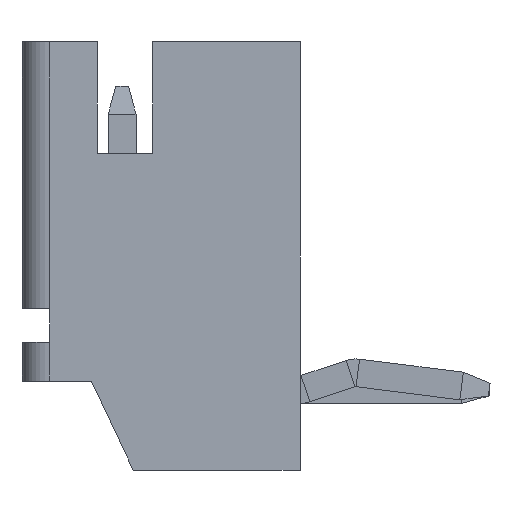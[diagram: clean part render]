
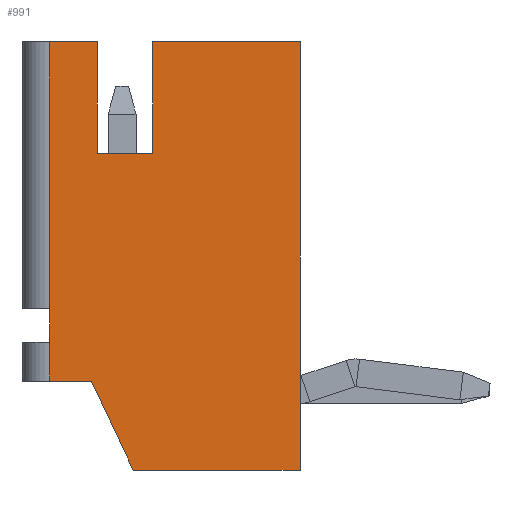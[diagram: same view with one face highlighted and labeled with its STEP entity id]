
A CAD part, left-side view. The second image highlights one B-rep face of the part: STEP entity #991.
In plain terms, the highlighted planar face has unit normal (-1, 0, 0).
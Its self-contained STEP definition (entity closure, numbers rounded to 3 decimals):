
#13 = CARTESIAN_POINT ( 'NONE',  ( -2., 1.3, 0. ) ) ;
#51 = VECTOR ( 'NONE', #4264, 1000. ) ;
#98 = CARTESIAN_POINT ( 'NONE',  ( -2., 1.3, 1.3 ) ) ;
#130 = EDGE_CURVE ( 'NONE', #6162, #6657, #4499, .T. ) ;
#144 = VERTEX_POINT ( 'NONE', #475 ) ;
#177 = CARTESIAN_POINT ( 'NONE',  ( -2., -3.2, -1.6 ) ) ;
#223 = ORIENTED_EDGE ( 'NONE', *, *, #1358, .T. ) ;
#278 = VECTOR ( 'NONE', #2242, 1000. ) ;
#312 = CARTESIAN_POINT ( 'NONE',  ( -2., 1.3, 6.1 ) ) ;
#313 = CARTESIAN_POINT ( 'NONE',  ( -2., 1.3, 1.3 ) ) ;
#388 = EDGE_LOOP ( 'NONE', ( #1018, #1633, #5628, #573, #6049, #5959, #5366, #223, #3068, #3339, #4665, #1681 ) ) ;
#448 = EDGE_CURVE ( 'NONE', #1024, #3373, #1513, .T. ) ;
#475 = CARTESIAN_POINT ( 'NONE',  ( -2., 0.55, 0. ) ) ;
#573 = ORIENTED_EDGE ( 'NONE', *, *, #1032, .T. ) ;
#593 = CARTESIAN_POINT ( 'NONE',  ( -2., 1.3, 0. ) ) ;
#616 = DIRECTION ( 'NONE',  ( 0., 0., -1. ) ) ;
#653 = CARTESIAN_POINT ( 'NONE',  ( -2., -3.2, 6.1 ) ) ;
#654 = CARTESIAN_POINT ( 'NONE',  ( -2., 1.3, 0.7 ) ) ;
#693 = VECTOR ( 'NONE', #4263, 1000. ) ;
#991 = ADVANCED_FACE ( 'NONE', ( #5384 ), #5811, .T. ) ;
#1018 = ORIENTED_EDGE ( 'NONE', *, *, #2460, .T. ) ;
#1024 = VERTEX_POINT ( 'NONE', #177 ) ;
#1032 = EDGE_CURVE ( 'NONE', #144, #1546, #3606, .T. ) ;
#1115 = VECTOR ( 'NONE', #4143, 1000. ) ;
#1137 = DIRECTION ( 'NONE',  ( -1., 0., 0. ) ) ;
#1193 = CARTESIAN_POINT ( 'NONE',  ( -2., 0.45, 4.1 ) ) ;
#1358 = EDGE_CURVE ( 'NONE', #1372, #6162, #3042, .T. ) ;
#1372 = VERTEX_POINT ( 'NONE', #2681 ) ;
#1513 = LINE ( 'NONE', #3240, #51 ) ;
#1518 = VECTOR ( 'NONE', #3710, 1000. ) ;
#1546 = VERTEX_POINT ( 'NONE', #2281 ) ;
#1588 = EDGE_CURVE ( 'NONE', #5779, #4288, #2639, .T. ) ;
#1633 = ORIENTED_EDGE ( 'NONE', *, *, #1588, .T. ) ;
#1656 = LINE ( 'NONE', #3238, #278 ) ;
#1678 = CARTESIAN_POINT ( 'NONE',  ( -2., -0.55, 6.1 ) ) ;
#1681 = ORIENTED_EDGE ( 'NONE', *, *, #1809, .T. ) ;
#1741 = DIRECTION ( 'NONE',  ( 0., -1., 0. ) ) ;
#1809 = EDGE_CURVE ( 'NONE', #3515, #5945, #3206, .T. ) ;
#1899 = CARTESIAN_POINT ( 'NONE',  ( -2., -0.55, 4.1 ) ) ;
#2242 = DIRECTION ( 'NONE',  ( 0., 1., 0. ) ) ;
#2281 = CARTESIAN_POINT ( 'NONE',  ( -2., -0.2, -1.6 ) ) ;
#2403 = DIRECTION ( 'NONE',  ( 0., 0., -1. ) ) ;
#2460 = EDGE_CURVE ( 'NONE', #5945, #5779, #3911, .T. ) ;
#2543 = VECTOR ( 'NONE', #3811, 1000. ) ;
#2548 = VECTOR ( 'NONE', #1741, 1000. ) ;
#2596 = DIRECTION ( 'NONE',  ( 0., 0., -1. ) ) ;
#2639 = LINE ( 'NONE', #2905, #5448 ) ;
#2681 = CARTESIAN_POINT ( 'NONE',  ( -2., -0.55, 6.1 ) ) ;
#2745 = DIRECTION ( 'NONE',  ( 0., -1., 0. ) ) ;
#2905 = CARTESIAN_POINT ( 'NONE',  ( -2., 1.3, 0. ) ) ;
#2951 = LINE ( 'NONE', #1678, #693 ) ;
#2964 = VECTOR ( 'NONE', #2596, 1000. ) ;
#3042 = LINE ( 'NONE', #4677, #6099 ) ;
#3068 = ORIENTED_EDGE ( 'NONE', *, *, #130, .T. ) ;
#3205 = CARTESIAN_POINT ( 'NONE',  ( -2., 1.8, 0. ) ) ;
#3206 = LINE ( 'NONE', #593, #2964 ) ;
#3238 = CARTESIAN_POINT ( 'NONE',  ( -2., 1.8, 6.1 ) ) ;
#3240 = CARTESIAN_POINT ( 'NONE',  ( -2., -3.2, 6.1 ) ) ;
#3339 = ORIENTED_EDGE ( 'NONE', *, *, #5858, .T. ) ;
#3373 = VERTEX_POINT ( 'NONE', #653 ) ;
#3515 = VERTEX_POINT ( 'NONE', #312 ) ;
#3606 = LINE ( 'NONE', #6324, #1518 ) ;
#3638 = DIRECTION ( 'NONE',  ( 0., -1., 0. ) ) ;
#3710 = DIRECTION ( 'NONE',  ( 0., -0.424, -0.905 ) ) ;
#3811 = DIRECTION ( 'NONE',  ( 0., 0., 1. ) ) ;
#3901 = LINE ( 'NONE', #5809, #2543 ) ;
#3911 = LINE ( 'NONE', #98, #4147 ) ;
#4064 = LINE ( 'NONE', #3205, #2548 ) ;
#4077 = CARTESIAN_POINT ( 'NONE',  ( -2., 0.45, 4.1 ) ) ;
#4143 = DIRECTION ( 'NONE',  ( 0., 1., 0. ) ) ;
#4147 = VECTOR ( 'NONE', #616, 1000. ) ;
#4180 = VERTEX_POINT ( 'NONE', #6006 ) ;
#4214 = CARTESIAN_POINT ( 'NONE',  ( -2., 0., 0. ) ) ;
#4263 = DIRECTION ( 'NONE',  ( 0., 1., 0. ) ) ;
#4264 = DIRECTION ( 'NONE',  ( 0., 0., 1. ) ) ;
#4288 = VERTEX_POINT ( 'NONE', #13 ) ;
#4368 = EDGE_CURVE ( 'NONE', #4288, #144, #4064, .T. ) ;
#4387 = VECTOR ( 'NONE', #3638, 1000. ) ;
#4499 = LINE ( 'NONE', #4077, #1115 ) ;
#4548 = AXIS2_PLACEMENT_3D ( 'NONE', #4214, #1137, #2745 ) ;
#4635 = LINE ( 'NONE', #4639, #4387 ) ;
#4639 = CARTESIAN_POINT ( 'NONE',  ( -2., -3.2, -1.6 ) ) ;
#4665 = ORIENTED_EDGE ( 'NONE', *, *, #5837, .T. ) ;
#4677 = CARTESIAN_POINT ( 'NONE',  ( -2., -0.55, 6.1 ) ) ;
#4732 = EDGE_CURVE ( 'NONE', #3373, #1372, #2951, .T. ) ;
#5366 = ORIENTED_EDGE ( 'NONE', *, *, #4732, .T. ) ;
#5384 = FACE_OUTER_BOUND ( 'NONE', #388, .T. ) ;
#5448 = VECTOR ( 'NONE', #2403, 1000. ) ;
#5480 = EDGE_CURVE ( 'NONE', #1546, #1024, #4635, .T. ) ;
#5628 = ORIENTED_EDGE ( 'NONE', *, *, #4368, .T. ) ;
#5779 = VERTEX_POINT ( 'NONE', #654 ) ;
#5809 = CARTESIAN_POINT ( 'NONE',  ( -2., 0.45, 6.1 ) ) ;
#5811 = PLANE ( 'NONE',  #4548 ) ;
#5837 = EDGE_CURVE ( 'NONE', #4180, #3515, #1656, .T. ) ;
#5858 = EDGE_CURVE ( 'NONE', #6657, #4180, #3901, .T. ) ;
#5945 = VERTEX_POINT ( 'NONE', #313 ) ;
#5959 = ORIENTED_EDGE ( 'NONE', *, *, #448, .T. ) ;
#6006 = CARTESIAN_POINT ( 'NONE',  ( -2., 0.45, 6.1 ) ) ;
#6049 = ORIENTED_EDGE ( 'NONE', *, *, #5480, .T. ) ;
#6099 = VECTOR ( 'NONE', #6246, 1000. ) ;
#6162 = VERTEX_POINT ( 'NONE', #1899 ) ;
#6246 = DIRECTION ( 'NONE',  ( 0., 0., -1. ) ) ;
#6324 = CARTESIAN_POINT ( 'NONE',  ( -2., -0.2, -1.6 ) ) ;
#6657 = VERTEX_POINT ( 'NONE', #1193 ) ;
